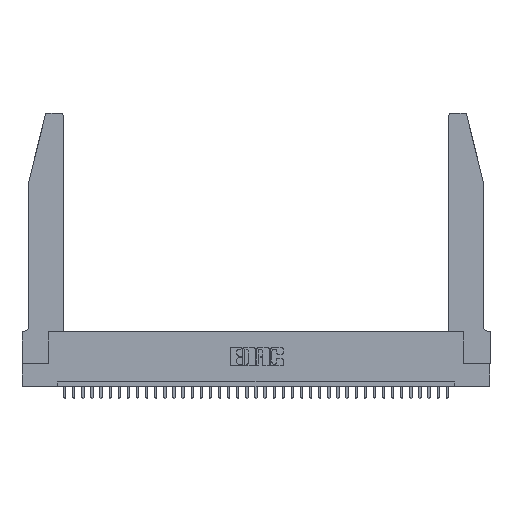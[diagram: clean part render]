
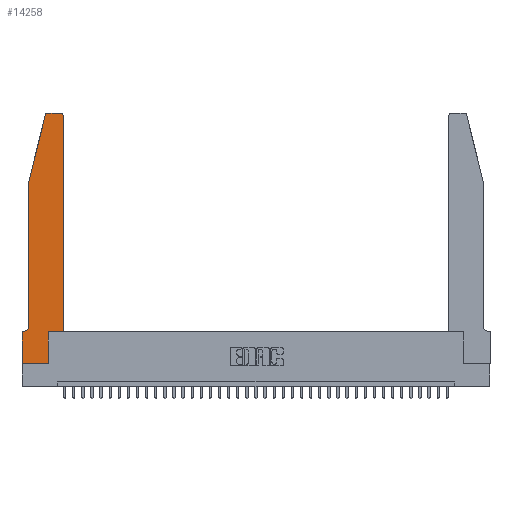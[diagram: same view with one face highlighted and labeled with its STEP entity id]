
A CAD part, top view. The second image highlights one B-rep face of the part: STEP entity #14258.
In plain terms, the highlighted planar face has unit normal (0, 0, 1).
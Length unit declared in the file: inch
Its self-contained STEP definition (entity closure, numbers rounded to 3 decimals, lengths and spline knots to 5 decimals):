
#28 = VECTOR ( 'NONE', #5467, 39.37008 ) ;
#30 = LINE ( 'NONE', #18968, #7094 ) ;
#425 = VERTEX_POINT ( 'NONE', #22414 ) ;
#719 = AXIS2_PLACEMENT_3D ( 'NONE', #3936, #17994, #23967 ) ;
#910 = AXIS2_PLACEMENT_3D ( 'NONE', #36188, #8042, #2808 ) ;
#1262 = CARTESIAN_POINT ( 'NONE',  ( 0., 0.35, 0.37 ) ) ;
#1293 = CARTESIAN_POINT ( 'NONE',  ( 0.4505, 2.72, 0.37 ) ) ;
#1569 = ORIENTED_EDGE ( 'NONE', *, *, #27459, .T. ) ;
#1577 = VERTEX_POINT ( 'NONE', #28847 ) ;
#1827 = CARTESIAN_POINT ( 'NONE',  ( 0.4505, 0.35, 0.37 ) ) ;
#1946 = EDGE_CURVE ( 'NONE', #14865, #26650, #27438, .T. ) ;
#2162 = EDGE_CURVE ( 'NONE', #35574, #31514, #30480, .T. ) ;
#2808 = DIRECTION ( 'NONE',  ( 1., 0., 0. ) ) ;
#2926 = FACE_OUTER_BOUND ( 'NONE', #15961, .T. ) ;
#3048 = DIRECTION ( 'NONE',  ( 0., 1., 0. ) ) ;
#3063 = CARTESIAN_POINT ( 'NONE',  ( 0., 0., 0.37 ) ) ;
#3255 = CARTESIAN_POINT ( 'NONE',  ( 0.4205, 2.75, 0.37 ) ) ;
#3511 = CARTESIAN_POINT ( 'NONE',  ( 0.25487, 2.72718, 0.37 ) ) ;
#3936 = CARTESIAN_POINT ( 'NONE',  ( 0.284, 2.72, 0.37 ) ) ;
#4303 = ORIENTED_EDGE ( 'NONE', *, *, #23715, .T. ) ;
#4394 = ORIENTED_EDGE ( 'NONE', *, *, #22974, .T. ) ;
#5467 = DIRECTION ( 'NONE',  ( 0., -1., 0. ) ) ;
#5660 = LINE ( 'NONE', #14664, #10548 ) ;
#5753 = CIRCLE ( 'NONE', #719, 0.03 ) ;
#5822 = DIRECTION ( 'NONE',  ( 1., 0., 0. ) ) ;
#5988 = CARTESIAN_POINT ( 'NONE',  ( 0.0755, 0.35, 0.37 ) ) ;
#6436 = CARTESIAN_POINT ( 'NONE',  ( 0.2865, 0., 0.37 ) ) ;
#7094 = VECTOR ( 'NONE', #27575, 39.37008 ) ;
#8042 = DIRECTION ( 'NONE',  ( 0., 0., 1. ) ) ;
#8149 = LINE ( 'NONE', #1827, #35882 ) ;
#8922 = CARTESIAN_POINT ( 'NONE',  ( 0.4505, 0.35, 0.37 ) ) ;
#9386 = EDGE_CURVE ( 'NONE', #21853, #425, #22799, .T. ) ;
#10466 = VECTOR ( 'NONE', #16995, 39.37008 ) ;
#10548 = VECTOR ( 'NONE', #34606, 39.37008 ) ;
#10671 = ORIENTED_EDGE ( 'NONE', *, *, #27507, .T. ) ;
#12661 = CARTESIAN_POINT ( 'NONE',  ( 0.0755, 2., 0.37 ) ) ;
#12926 = VECTOR ( 'NONE', #5822, 39.37008 ) ;
#13865 = CARTESIAN_POINT ( 'NONE',  ( 0.0055, 0.35, 0.37 ) ) ;
#13885 = DIRECTION ( 'NONE',  ( 0., -1., 0. ) ) ;
#13888 = AXIS2_PLACEMENT_3D ( 'NONE', #36488, #22558, #31131 ) ;
#14258 = ADVANCED_FACE ( 'NONE', ( #2926 ), #33295, .T. ) ;
#14423 = CARTESIAN_POINT ( 'NONE',  ( 0.2605, 2.75, 0.37 ) ) ;
#14563 = DIRECTION ( 'NONE',  ( 0., 0., -1. ) ) ;
#14664 = CARTESIAN_POINT ( 'NONE',  ( 0., 0., 0.37 ) ) ;
#14865 = VERTEX_POINT ( 'NONE', #1262 ) ;
#15958 = ORIENTED_EDGE ( 'NONE', *, *, #1946, .T. ) ;
#15961 = EDGE_LOOP ( 'NONE', ( #1569, #23748, #4394, #33839, #30660, #32254, #15958, #10671, #36218, #21535, #19529, #4303 ) ) ;
#16023 = EDGE_CURVE ( 'NONE', #425, #26932, #8149, .T. ) ;
#16995 = DIRECTION ( 'NONE',  ( 0., 1., 0. ) ) ;
#17187 = DIRECTION ( 'NONE',  ( -1., 0., 0. ) ) ;
#17994 = DIRECTION ( 'NONE',  ( 0., 0., 1. ) ) ;
#18968 = CARTESIAN_POINT ( 'NONE',  ( 0.0755, 2., 0.37 ) ) ;
#19529 = ORIENTED_EDGE ( 'NONE', *, *, #16023, .T. ) ;
#20300 = CARTESIAN_POINT ( 'NONE',  ( 0., 0., 0.37 ) ) ;
#20328 = DIRECTION ( 'NONE',  ( -1., 0., 0. ) ) ;
#21535 = ORIENTED_EDGE ( 'NONE', *, *, #9386, .T. ) ;
#21853 = VERTEX_POINT ( 'NONE', #24483 ) ;
#22044 = VERTEX_POINT ( 'NONE', #3255 ) ;
#22286 = LINE ( 'NONE', #14423, #23616 ) ;
#22414 = CARTESIAN_POINT ( 'NONE',  ( 0.4505, 0.35, 0.37 ) ) ;
#22558 = DIRECTION ( 'NONE',  ( 0., 0., 1. ) ) ;
#22799 = LINE ( 'NONE', #8922, #12926 ) ;
#22974 = EDGE_CURVE ( 'NONE', #27638, #35020, #30, .T. ) ;
#23616 = VECTOR ( 'NONE', #17187, 39.37008 ) ;
#23715 = EDGE_CURVE ( 'NONE', #26932, #22044, #26202, .T. ) ;
#23748 = ORIENTED_EDGE ( 'NONE', *, *, #26400, .T. ) ;
#23967 = DIRECTION ( 'NONE',  ( 1., 0., 0. ) ) ;
#24308 = VECTOR ( 'NONE', #26657, 39.37008 ) ;
#24483 = CARTESIAN_POINT ( 'NONE',  ( 0.2865, 0.35, 0.37 ) ) ;
#24535 = VERTEX_POINT ( 'NONE', #6436 ) ;
#25080 = EDGE_CURVE ( 'NONE', #31514, #14865, #36793, .T. ) ;
#25622 = CARTESIAN_POINT ( 'NONE',  ( 0.0755, 2., 0.37 ) ) ;
#26202 = CIRCLE ( 'NONE', #13888, 0.03 ) ;
#26400 = EDGE_CURVE ( 'NONE', #1577, #27638, #5753, .T. ) ;
#26650 = VERTEX_POINT ( 'NONE', #3063 ) ;
#26657 = DIRECTION ( 'NONE',  ( -1., 0., 0. ) ) ;
#26932 = VERTEX_POINT ( 'NONE', #1293 ) ;
#27438 = LINE ( 'NONE', #20300, #36313 ) ;
#27459 = EDGE_CURVE ( 'NONE', #22044, #1577, #22286, .T. ) ;
#27507 = EDGE_CURVE ( 'NONE', #26650, #24535, #5660, .T. ) ;
#27575 = DIRECTION ( 'NONE',  ( -0.239, -0.971, 0. ) ) ;
#27638 = VERTEX_POINT ( 'NONE', #3511 ) ;
#28235 = CARTESIAN_POINT ( 'NONE',  ( 0.2865, 0.35, 0.37 ) ) ;
#28445 = CARTESIAN_POINT ( 'NONE',  ( 0.0055, 0.42, 0.37 ) ) ;
#28847 = CARTESIAN_POINT ( 'NONE',  ( 0.284, 2.75, 0.37 ) ) ;
#30480 = CIRCLE ( 'NONE', #30541, 0.07 ) ;
#30541 = AXIS2_PLACEMENT_3D ( 'NONE', #28445, #14563, #20328 ) ;
#30660 = ORIENTED_EDGE ( 'NONE', *, *, #2162, .T. ) ;
#31131 = DIRECTION ( 'NONE',  ( 1., 0., 0. ) ) ;
#31514 = VERTEX_POINT ( 'NONE', #13865 ) ;
#31568 = EDGE_CURVE ( 'NONE', #35020, #35574, #32200, .T. ) ;
#32200 = LINE ( 'NONE', #25622, #28 ) ;
#32254 = ORIENTED_EDGE ( 'NONE', *, *, #25080, .T. ) ;
#32858 = LINE ( 'NONE', #28235, #10466 ) ;
#33295 = PLANE ( 'NONE',  #910 ) ;
#33626 = EDGE_CURVE ( 'NONE', #24535, #21853, #32858, .T. ) ;
#33839 = ORIENTED_EDGE ( 'NONE', *, *, #31568, .T. ) ;
#34606 = DIRECTION ( 'NONE',  ( 1., 0., 0. ) ) ;
#35020 = VERTEX_POINT ( 'NONE', #12661 ) ;
#35574 = VERTEX_POINT ( 'NONE', #36739 ) ;
#35882 = VECTOR ( 'NONE', #3048, 39.37008 ) ;
#36188 = CARTESIAN_POINT ( 'NONE',  ( 0., 0.35, 0.37 ) ) ;
#36218 = ORIENTED_EDGE ( 'NONE', *, *, #33626, .T. ) ;
#36313 = VECTOR ( 'NONE', #13885, 39.37008 ) ;
#36488 = CARTESIAN_POINT ( 'NONE',  ( 0.4205, 2.72, 0.37 ) ) ;
#36739 = CARTESIAN_POINT ( 'NONE',  ( 0.0755, 0.42, 0.37 ) ) ;
#36793 = LINE ( 'NONE', #5988, #24308 ) ;
